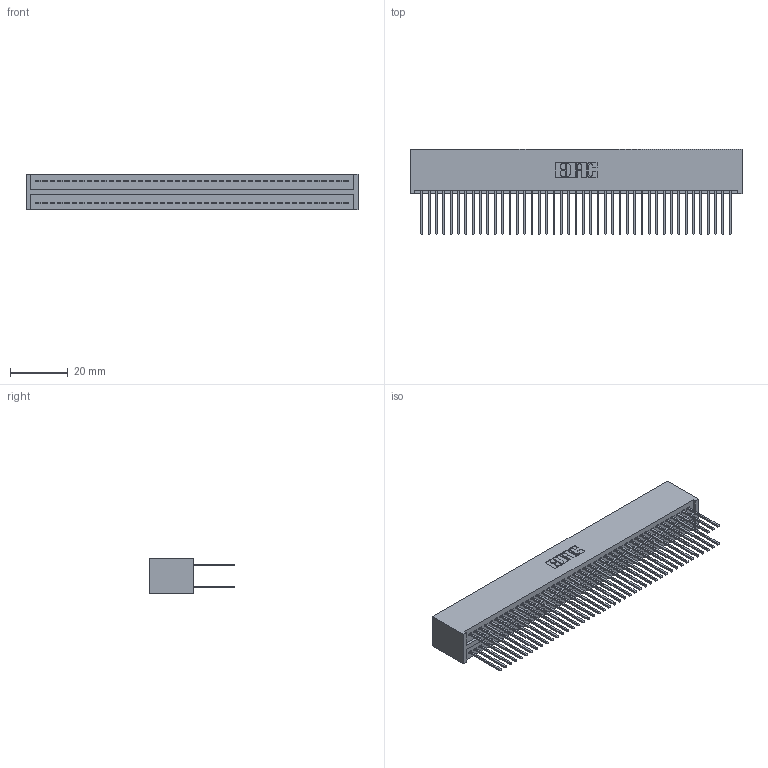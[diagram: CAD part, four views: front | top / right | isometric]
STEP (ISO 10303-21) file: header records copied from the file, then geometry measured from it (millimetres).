
FILE_DESCRIPTION (( 'STEP AP203' ), '1' );
FILE_NAME ('325-086-540-201.STEP', '2020-02-25T05:16:51', ( '' ), ( '' ), 'SwSTEP 2.0', 'SolidWorks 2016', '' );
FILE_SCHEMA (( 'CONFIG_CONTROL_DESIGN' ));
Length unit declared in the file: inch
Products named in the file (3): 325 Part_Lugless; 325-292-001_325-293-140; 325-086-540-201
Assembly tree (87 placements, depth 2):
  325-086-540-201
    325 Part_Lugless
    325-292-001_325-293-140  x86
Bounding box: 114.86 x 29.46 x 12.45 mm (x, y, z)
Volume: 15769.1 mm3; surface area: 21323.1 mm2
Topology: 87 solids, 87 shells, 4578 faces, 13617 edges, 8962 vertices
Faces by surface type: plane 3162, cylinder 1416
Entity records: 27275 total; most frequent: CARTESIAN_POINT 4518, ORIENTED_EDGE 4454, DIRECTION 3851, EDGE_CURVE 2227, LINE 2107, VECTOR 2107, VERTEX_POINT 1482, AXIS2_PLACEMENT_3D 872
